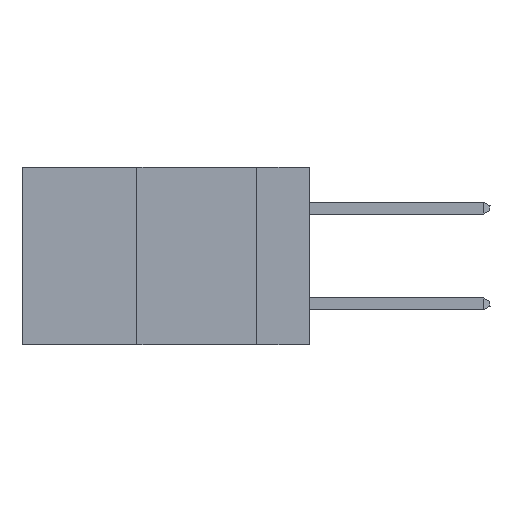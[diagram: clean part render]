
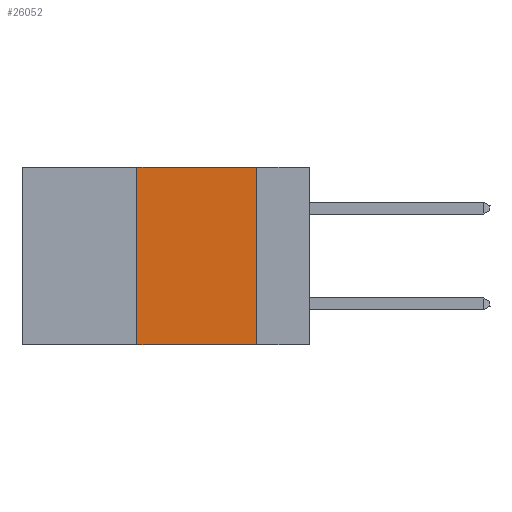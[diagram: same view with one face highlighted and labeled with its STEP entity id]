
A CAD part, left-side view. The second image highlights one B-rep face of the part: STEP entity #26052.
In plain terms, the highlighted planar face has unit normal (-1, 0, 0).
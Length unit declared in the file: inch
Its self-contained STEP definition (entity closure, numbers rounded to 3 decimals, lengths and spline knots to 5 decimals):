
#2189 = LINE ( 'NONE', #32331, #9646 ) ;
#2265 = EDGE_CURVE ( 'NONE', #17132, #30465, #23661, .T. ) ;
#2642 = CARTESIAN_POINT ( 'NONE',  ( 0., 0.36, -0.37 ) ) ;
#3502 = EDGE_CURVE ( 'NONE', #11995, #17132, #2189, .T. ) ;
#5166 = CARTESIAN_POINT ( 'NONE',  ( 0., 0.6, 0. ) ) ;
#5511 = CARTESIAN_POINT ( 'NONE',  ( 0., 0.11, -0.37 ) ) ;
#7103 = CARTESIAN_POINT ( 'NONE',  ( 0., 0.6, -0.37 ) ) ;
#7523 = VECTOR ( 'NONE', #21643, 39.37008 ) ;
#8889 = EDGE_CURVE ( 'NONE', #31067, #30465, #36795, .T. ) ;
#9646 = VECTOR ( 'NONE', #16311, 39.37008 ) ;
#11070 = CARTESIAN_POINT ( 'NONE',  ( 0., 0.11, 0. ) ) ;
#11214 = CARTESIAN_POINT ( 'NONE',  ( 0., 0.36, 0. ) ) ;
#11508 = DIRECTION ( 'NONE',  ( 0., 0., -1. ) ) ;
#11995 = VERTEX_POINT ( 'NONE', #11214 ) ;
#12849 = ORIENTED_EDGE ( 'NONE', *, *, #16838, .F. ) ;
#13785 = DIRECTION ( 'NONE',  ( 0., -1., 0. ) ) ;
#14897 = PLANE ( 'NONE',  #31093 ) ;
#15629 = VECTOR ( 'NONE', #11508, 39.37008 ) ;
#16311 = DIRECTION ( 'NONE',  ( 0., -1., 0. ) ) ;
#16838 = EDGE_CURVE ( 'NONE', #31067, #11995, #40097, .T. ) ;
#17132 = VERTEX_POINT ( 'NONE', #11070 ) ;
#18196 = ORIENTED_EDGE ( 'NONE', *, *, #2265, .F. ) ;
#21643 = DIRECTION ( 'NONE',  ( 0., 0., 1. ) ) ;
#22429 = ORIENTED_EDGE ( 'NONE', *, *, #3502, .F. ) ;
#23661 = LINE ( 'NONE', #37480, #15629 ) ;
#26052 = ADVANCED_FACE ( 'NONE', ( #36173 ), #14897, .F. ) ;
#27546 = DIRECTION ( 'NONE',  ( 1., 0., 0. ) ) ;
#28931 = EDGE_LOOP ( 'NONE', ( #18196, #22429, #12849, #38088 ) ) ;
#30465 = VERTEX_POINT ( 'NONE', #5511 ) ;
#31067 = VERTEX_POINT ( 'NONE', #2642 ) ;
#31093 = AXIS2_PLACEMENT_3D ( 'NONE', #5166, #27546, #40037 ) ;
#31895 = CARTESIAN_POINT ( 'NONE',  ( 0., 0.36, 0. ) ) ;
#32331 = CARTESIAN_POINT ( 'NONE',  ( 0., 0.6, 0. ) ) ;
#36173 = FACE_OUTER_BOUND ( 'NONE', #28931, .T. ) ;
#36795 = LINE ( 'NONE', #7103, #40769 ) ;
#37480 = CARTESIAN_POINT ( 'NONE',  ( 0., 0.11, 0. ) ) ;
#38088 = ORIENTED_EDGE ( 'NONE', *, *, #8889, .T. ) ;
#40037 = DIRECTION ( 'NONE',  ( 0., 0., -1. ) ) ;
#40097 = LINE ( 'NONE', #31895, #7523 ) ;
#40769 = VECTOR ( 'NONE', #13785, 39.37008 ) ;
